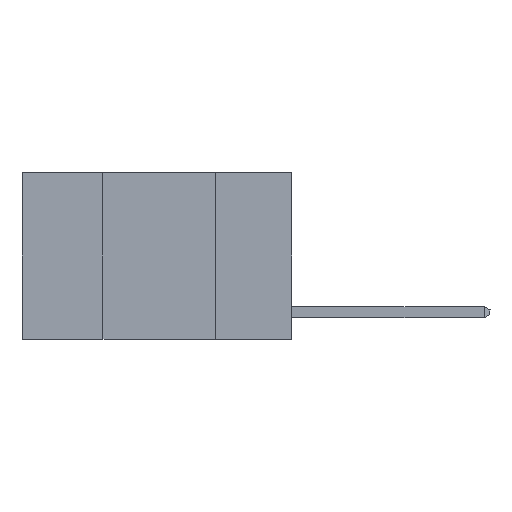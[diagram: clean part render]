
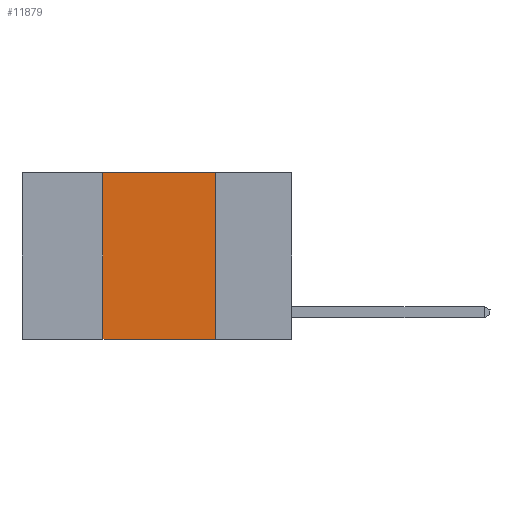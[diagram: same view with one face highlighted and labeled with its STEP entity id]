
A CAD part, left-side view. The second image highlights one B-rep face of the part: STEP entity #11879.
In plain terms, the highlighted planar face has unit normal (-1, 0, 0).
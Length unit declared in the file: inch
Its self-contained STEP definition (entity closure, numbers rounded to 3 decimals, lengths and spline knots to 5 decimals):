
#126 = CARTESIAN_POINT ( 'NONE',  ( 0., 0.42, 0. ) ) ;
#1417 = ORIENTED_EDGE ( 'NONE', *, *, #9623, .F. ) ;
#2027 = LINE ( 'NONE', #13631, #16477 ) ;
#2247 = DIRECTION ( 'NONE',  ( 0., 0., 1. ) ) ;
#2659 = EDGE_CURVE ( 'NONE', #16548, #13043, #16508, .T. ) ;
#2873 = DIRECTION ( 'NONE',  ( 0., -1., 0. ) ) ;
#3021 = PLANE ( 'NONE',  #11704 ) ;
#3062 = EDGE_CURVE ( 'NONE', #16484, #21767, #2027, .T. ) ;
#4060 = EDGE_CURVE ( 'NONE', #16548, #16484, #24570, .T. ) ;
#5106 = DIRECTION ( 'NONE',  ( 1., 0., 0. ) ) ;
#5487 = DIRECTION ( 'NONE',  ( 0., -1., 0. ) ) ;
#6983 = CARTESIAN_POINT ( 'NONE',  ( 0., 0.17, -0.37 ) ) ;
#9205 = CARTESIAN_POINT ( 'NONE',  ( 0., 0.17, 0. ) ) ;
#9623 = EDGE_CURVE ( 'NONE', #21767, #13043, #14724, .T. ) ;
#11227 = DIRECTION ( 'NONE',  ( 0., 0., -1. ) ) ;
#11704 = AXIS2_PLACEMENT_3D ( 'NONE', #17347, #5106, #19352 ) ;
#11879 = ADVANCED_FACE ( 'NONE', ( #23401 ), #3021, .F. ) ;
#13043 = VERTEX_POINT ( 'NONE', #6983 ) ;
#13631 = CARTESIAN_POINT ( 'NONE',  ( 0., 0.6, 0. ) ) ;
#14724 = LINE ( 'NONE', #9205, #24769 ) ;
#15172 = CARTESIAN_POINT ( 'NONE',  ( 0., 0.6, -0.37 ) ) ;
#16301 = ORIENTED_EDGE ( 'NONE', *, *, #4060, .F. ) ;
#16477 = VECTOR ( 'NONE', #5487, 39.37008 ) ;
#16484 = VERTEX_POINT ( 'NONE', #17348 ) ;
#16508 = LINE ( 'NONE', #15172, #21207 ) ;
#16548 = VERTEX_POINT ( 'NONE', #25585 ) ;
#17347 = CARTESIAN_POINT ( 'NONE',  ( 0., 0.6, 0. ) ) ;
#17348 = CARTESIAN_POINT ( 'NONE',  ( 0., 0.42, 0. ) ) ;
#19352 = DIRECTION ( 'NONE',  ( 0., 0., -1. ) ) ;
#19560 = EDGE_LOOP ( 'NONE', ( #1417, #21738, #16301, #22045 ) ) ;
#19883 = VECTOR ( 'NONE', #2247, 39.37008 ) ;
#21207 = VECTOR ( 'NONE', #2873, 39.37008 ) ;
#21738 = ORIENTED_EDGE ( 'NONE', *, *, #3062, .F. ) ;
#21767 = VERTEX_POINT ( 'NONE', #23830 ) ;
#22045 = ORIENTED_EDGE ( 'NONE', *, *, #2659, .T. ) ;
#23401 = FACE_OUTER_BOUND ( 'NONE', #19560, .T. ) ;
#23830 = CARTESIAN_POINT ( 'NONE',  ( 0., 0.17, 0. ) ) ;
#24570 = LINE ( 'NONE', #126, #19883 ) ;
#24769 = VECTOR ( 'NONE', #11227, 39.37008 ) ;
#25585 = CARTESIAN_POINT ( 'NONE',  ( 0., 0.42, -0.37 ) ) ;
